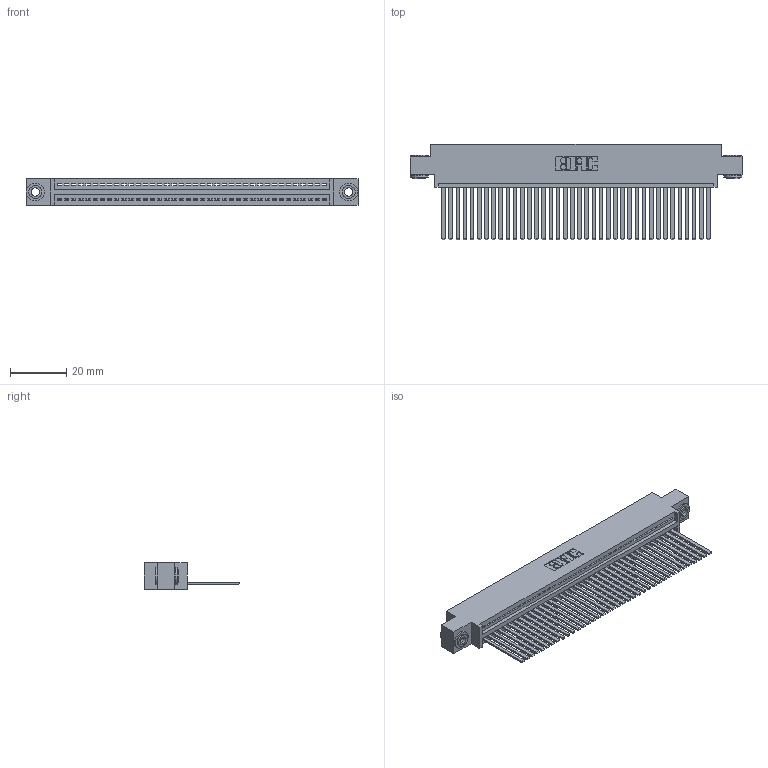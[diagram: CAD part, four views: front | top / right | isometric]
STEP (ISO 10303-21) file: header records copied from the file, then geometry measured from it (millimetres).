
FILE_DESCRIPTION (( 'STEP AP203' ), '1' );
FILE_NAME ('345-038-544-603.STEP', '2018-08-30T09:03:09', ( '' ), ( '' ), 'SwSTEP 2.0', 'SolidWorks 2016', '' );
FILE_SCHEMA (( 'CONFIG_CONTROL_DESIGN' ));
Length unit declared in the file: inch
Products named in the file (4): 345 Part_0.170 Offset - 0.156 Dia-TH; 345-292-001_345-293-144; 345-250-002_345-250-002-102; 345-038-544-603
Assembly tree (41 placements, depth 2):
  345-038-544-603
    345 Part_0.170 Offset - 0.156 Dia-TH
    345-292-001_345-293-144  x38
    345-250-002_345-250-002-102  x2
Bounding box: 117.73 x 33.96 x 9.4 mm (x, y, z)
Volume: 11495.4 mm3; surface area: 16884.2 mm2
Topology: 41 solids, 41 shells, 2144 faces, 6433 edges, 4234 vertices
Faces by surface type: plane 1462, cylinder 674, cone 8
Entity records: 29736 total; most frequent: CARTESIAN_POINT 5129, ORIENTED_EDGE 5094, DIRECTION 4513, EDGE_CURVE 2547, VECTOR 2243, LINE 2243, VERTEX_POINT 1694, AXIS2_PLACEMENT_3D 1135
